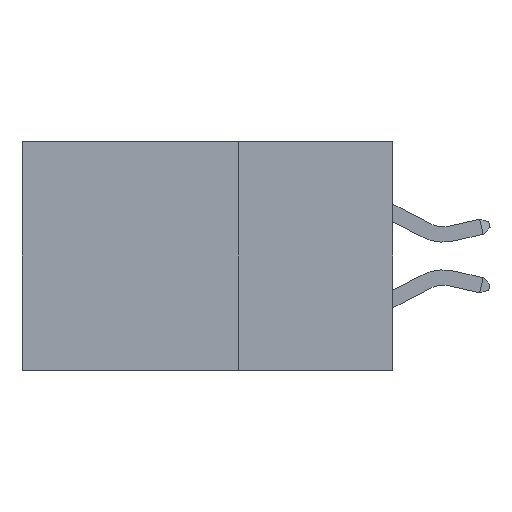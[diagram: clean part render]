
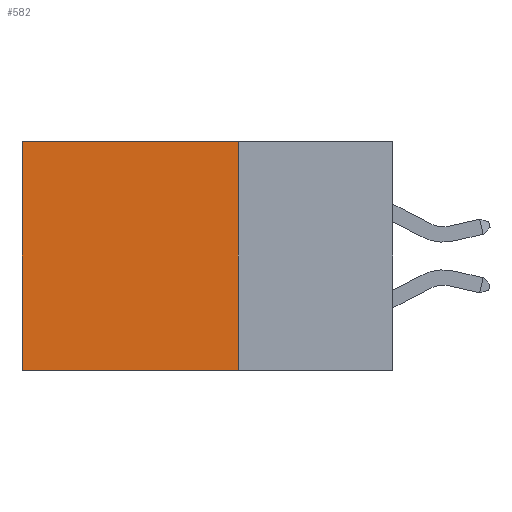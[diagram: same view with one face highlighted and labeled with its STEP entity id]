
A CAD part, left-side view. The second image highlights one B-rep face of the part: STEP entity #582.
In plain terms, the highlighted planar face has unit normal (-1, 0, 0).
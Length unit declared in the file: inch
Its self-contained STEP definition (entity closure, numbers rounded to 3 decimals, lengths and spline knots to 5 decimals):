
#276 = CARTESIAN_POINT ( 'NONE',  ( 0.2875, 0.6, 0. ) ) ;
#582 = ADVANCED_FACE ( 'NONE', ( #9615 ), #25695, .F. ) ;
#834 = DIRECTION ( 'NONE',  ( 0., 0., -1. ) ) ;
#1179 = ORIENTED_EDGE ( 'NONE', *, *, #23589, .T. ) ;
#1394 = EDGE_CURVE ( 'NONE', #25808, #18355, #23300, .T. ) ;
#3614 = LINE ( 'NONE', #11577, #11185 ) ;
#5286 = CARTESIAN_POINT ( 'NONE',  ( 0.2875, 0.6, -0.37 ) ) ;
#5502 = VECTOR ( 'NONE', #11973, 39.37008 ) ;
#5617 = EDGE_CURVE ( 'NONE', #25808, #6963, #7670, .T. ) ;
#5719 = CARTESIAN_POINT ( 'NONE',  ( 0.2875, 0.25, 0. ) ) ;
#5775 = DIRECTION ( 'NONE',  ( 0., 0., -1. ) ) ;
#6598 = VERTEX_POINT ( 'NONE', #5286 ) ;
#6963 = VERTEX_POINT ( 'NONE', #276 ) ;
#7670 = LINE ( 'NONE', #13698, #5502 ) ;
#9294 = ORIENTED_EDGE ( 'NONE', *, *, #12485, .F. ) ;
#9615 = FACE_OUTER_BOUND ( 'NONE', #17029, .T. ) ;
#9870 = DIRECTION ( 'NONE',  ( 0., 0., -1. ) ) ;
#9998 = DIRECTION ( 'NONE',  ( 1., 0., 0. ) ) ;
#11185 = VECTOR ( 'NONE', #23607, 39.37008 ) ;
#11493 = VECTOR ( 'NONE', #5775, 39.37008 ) ;
#11577 = CARTESIAN_POINT ( 'NONE',  ( 0.2875, 0.25, -0.37 ) ) ;
#11973 = DIRECTION ( 'NONE',  ( 0., 1., 0. ) ) ;
#12485 = EDGE_CURVE ( 'NONE', #18355, #6598, #3614, .T. ) ;
#12763 = CARTESIAN_POINT ( 'NONE',  ( 0.2875, 0.6, 0. ) ) ;
#13223 = CARTESIAN_POINT ( 'NONE',  ( 0.2875, 0.25, 0. ) ) ;
#13591 = ORIENTED_EDGE ( 'NONE', *, *, #5617, .T. ) ;
#13698 = CARTESIAN_POINT ( 'NONE',  ( 0.2875, 0.25, 0. ) ) ;
#15245 = LINE ( 'NONE', #12763, #16015 ) ;
#16015 = VECTOR ( 'NONE', #834, 39.37008 ) ;
#17029 = EDGE_LOOP ( 'NONE', ( #1179, #9294, #22151, #13591 ) ) ;
#18355 = VERTEX_POINT ( 'NONE', #23678 ) ;
#20148 = AXIS2_PLACEMENT_3D ( 'NONE', #5719, #9998, #9870 ) ;
#21489 = CARTESIAN_POINT ( 'NONE',  ( 0.2875, 0.25, 0. ) ) ;
#22151 = ORIENTED_EDGE ( 'NONE', *, *, #1394, .F. ) ;
#23300 = LINE ( 'NONE', #21489, #11493 ) ;
#23589 = EDGE_CURVE ( 'NONE', #6963, #6598, #15245, .T. ) ;
#23607 = DIRECTION ( 'NONE',  ( 0., 1., 0. ) ) ;
#23678 = CARTESIAN_POINT ( 'NONE',  ( 0.2875, 0.25, -0.37 ) ) ;
#25695 = PLANE ( 'NONE',  #20148 ) ;
#25808 = VERTEX_POINT ( 'NONE', #13223 ) ;
